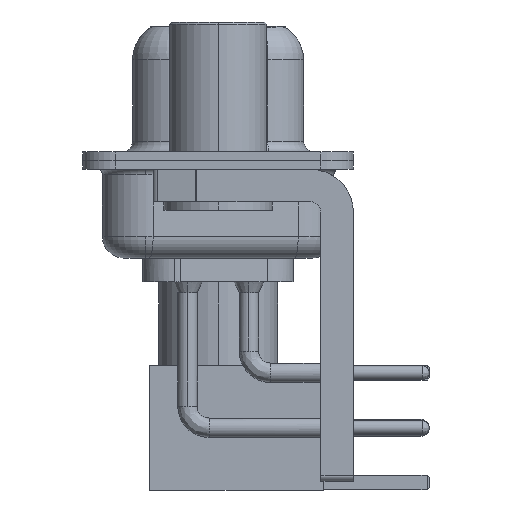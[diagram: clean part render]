
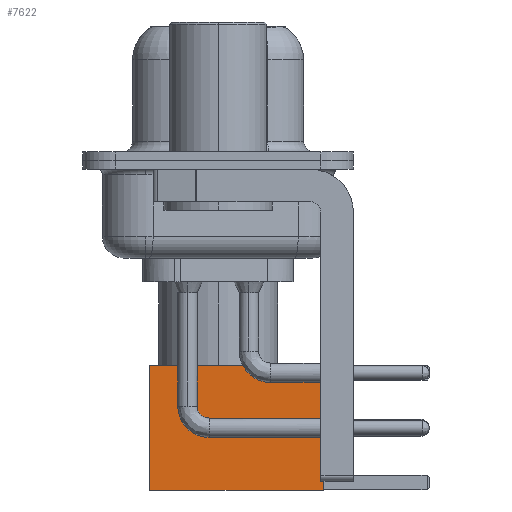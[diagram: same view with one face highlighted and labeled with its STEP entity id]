
A CAD part, left-side view. The second image highlights one B-rep face of the part: STEP entity #7622.
In plain terms, the highlighted face is planar.
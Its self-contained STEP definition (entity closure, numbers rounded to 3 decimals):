
#190 = DIRECTION ( 'NONE',  ( -1., 0., 0. ) ) ;
#702 = AXIS2_PLACEMENT_3D ( 'NONE', #9664, #21900, #3855 ) ;
#1248 = VERTEX_POINT ( 'NONE', #2958 ) ;
#2585 = DIRECTION ( 'NONE',  ( 0., 0., -1. ) ) ;
#2833 = CARTESIAN_POINT ( 'NONE',  ( 2.875, 2.875, 0. ) ) ;
#2958 = CARTESIAN_POINT ( 'NONE',  ( -2.875, 2.875, 0. ) ) ;
#3855 = DIRECTION ( 'NONE',  ( 0., 0., 1. ) ) ;
#4109 = ORIENTED_EDGE ( 'NONE', *, *, #10832, .T. ) ;
#5226 = VERTEX_POINT ( 'NONE', #15680 ) ;
#6167 = PLANE ( 'NONE',  #702 ) ;
#6591 = VERTEX_POINT ( 'NONE', #25364 ) ;
#6932 = CARTESIAN_POINT ( 'NONE',  ( 0., 2.875, 8. ) ) ;
#7622 = ADVANCED_FACE ( 'NONE', ( #23848 ), #6167, .T. ) ;
#9664 = CARTESIAN_POINT ( 'NONE',  ( 2.875, 2.875, 0. ) ) ;
#10328 = CARTESIAN_POINT ( 'NONE',  ( -2.875, 2.875, 0. ) ) ;
#10682 = CARTESIAN_POINT ( 'NONE',  ( 2.875, 2.875, 0. ) ) ;
#10832 = EDGE_CURVE ( 'NONE', #14569, #1248, #22859, .T. ) ;
#12380 = EDGE_LOOP ( 'NONE', ( #22382, #4109, #18419, #23333 ) ) ;
#14338 = LINE ( 'NONE', #2833, #24299 ) ;
#14569 = VERTEX_POINT ( 'NONE', #10682 ) ;
#15680 = CARTESIAN_POINT ( 'NONE',  ( 2.875, 2.875, 8. ) ) ;
#15879 = EDGE_CURVE ( 'NONE', #6591, #1248, #20246, .T. ) ;
#16514 = EDGE_CURVE ( 'NONE', #5226, #6591, #18563, .T. ) ;
#18419 = ORIENTED_EDGE ( 'NONE', *, *, #15879, .F. ) ;
#18563 = LINE ( 'NONE', #6932, #18776 ) ;
#18776 = VECTOR ( 'NONE', #18809, 1000. ) ;
#18809 = DIRECTION ( 'NONE',  ( -1., 0., 0. ) ) ;
#19794 = CARTESIAN_POINT ( 'NONE',  ( 0., 2.875, 0. ) ) ;
#20115 = DIRECTION ( 'NONE',  ( 0., 0., -1. ) ) ;
#20246 = LINE ( 'NONE', #10328, #23677 ) ;
#21214 = EDGE_CURVE ( 'NONE', #5226, #14569, #14338, .T. ) ;
#21900 = DIRECTION ( 'NONE',  ( 0., 1., 0. ) ) ;
#22382 = ORIENTED_EDGE ( 'NONE', *, *, #21214, .T. ) ;
#22859 = LINE ( 'NONE', #19794, #23325 ) ;
#23325 = VECTOR ( 'NONE', #190, 1000. ) ;
#23333 = ORIENTED_EDGE ( 'NONE', *, *, #16514, .F. ) ;
#23677 = VECTOR ( 'NONE', #2585, 1000. ) ;
#23848 = FACE_OUTER_BOUND ( 'NONE', #12380, .T. ) ;
#24299 = VECTOR ( 'NONE', #20115, 1000. ) ;
#25364 = CARTESIAN_POINT ( 'NONE',  ( -2.875, 2.875, 8. ) ) ;
